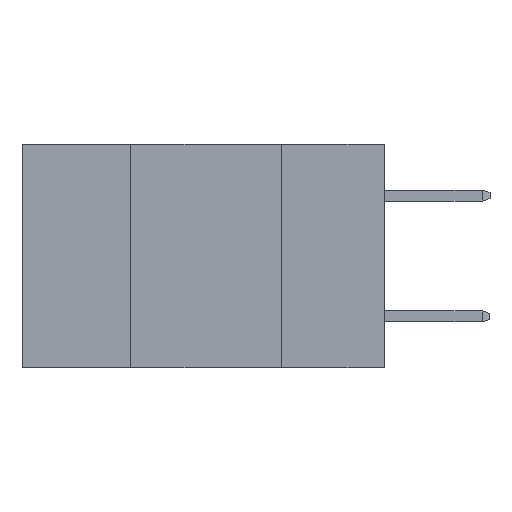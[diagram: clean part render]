
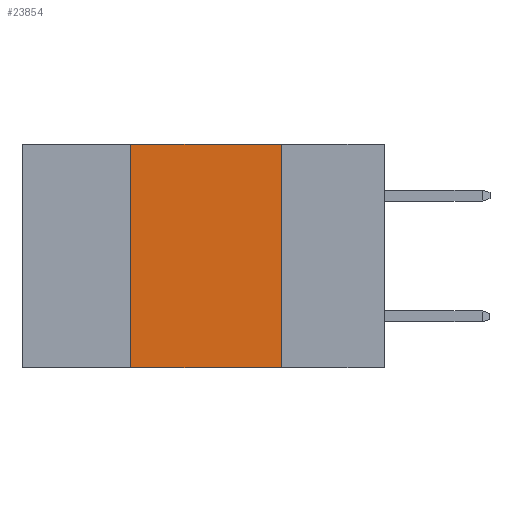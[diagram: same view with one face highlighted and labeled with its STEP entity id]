
A CAD part, left-side view. The second image highlights one B-rep face of the part: STEP entity #23854.
In plain terms, the highlighted planar face has unit normal (-1, 0, 0).
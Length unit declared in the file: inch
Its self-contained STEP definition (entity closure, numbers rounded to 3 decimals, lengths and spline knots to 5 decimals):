
#1426 = AXIS2_PLACEMENT_3D ( 'NONE', #3676, #22926, #11557 ) ;
#3478 = ORIENTED_EDGE ( 'NONE', *, *, #15090, .F. ) ;
#3676 = CARTESIAN_POINT ( 'NONE',  ( 0., 0.6, 0. ) ) ;
#3815 = DIRECTION ( 'NONE',  ( 0., 0., 1. ) ) ;
#3832 = LINE ( 'NONE', #7844, #13610 ) ;
#4682 = VERTEX_POINT ( 'NONE', #17868 ) ;
#4720 = VERTEX_POINT ( 'NONE', #16121 ) ;
#5701 = VERTEX_POINT ( 'NONE', #13211 ) ;
#6736 = VECTOR ( 'NONE', #3815, 39.37008 ) ;
#7844 = CARTESIAN_POINT ( 'NONE',  ( 0., 0.6, -0.37 ) ) ;
#8350 = CARTESIAN_POINT ( 'NONE',  ( 0., 0.17, 0. ) ) ;
#8696 = EDGE_LOOP ( 'NONE', ( #3478, #14446, #9935, #15042 ) ) ;
#8722 = CARTESIAN_POINT ( 'NONE',  ( 0., 0.6, 0. ) ) ;
#9371 = VECTOR ( 'NONE', #10516, 39.37008 ) ;
#9935 = ORIENTED_EDGE ( 'NONE', *, *, #16327, .F. ) ;
#10516 = DIRECTION ( 'NONE',  ( 0., -1., 0. ) ) ;
#11557 = DIRECTION ( 'NONE',  ( 0., 0., -1. ) ) ;
#12498 = LINE ( 'NONE', #22907, #6736 ) ;
#12610 = CARTESIAN_POINT ( 'NONE',  ( 0., 0.17, 0. ) ) ;
#13194 = EDGE_CURVE ( 'NONE', #4682, #13758, #19526, .T. ) ;
#13211 = CARTESIAN_POINT ( 'NONE',  ( 0., 0.42, -0.37 ) ) ;
#13610 = VECTOR ( 'NONE', #23116, 39.37008 ) ;
#13758 = VERTEX_POINT ( 'NONE', #8350 ) ;
#14446 = ORIENTED_EDGE ( 'NONE', *, *, #13194, .F. ) ;
#15042 = ORIENTED_EDGE ( 'NONE', *, *, #18908, .T. ) ;
#15090 = EDGE_CURVE ( 'NONE', #13758, #4720, #20318, .T. ) ;
#15277 = VECTOR ( 'NONE', #23948, 39.37008 ) ;
#16121 = CARTESIAN_POINT ( 'NONE',  ( 0., 0.17, -0.37 ) ) ;
#16327 = EDGE_CURVE ( 'NONE', #5701, #4682, #12498, .T. ) ;
#17868 = CARTESIAN_POINT ( 'NONE',  ( 0., 0.42, 0. ) ) ;
#18908 = EDGE_CURVE ( 'NONE', #5701, #4720, #3832, .T. ) ;
#19146 = PLANE ( 'NONE',  #1426 ) ;
#19526 = LINE ( 'NONE', #8722, #9371 ) ;
#20318 = LINE ( 'NONE', #12610, #15277 ) ;
#20876 = FACE_OUTER_BOUND ( 'NONE', #8696, .T. ) ;
#22907 = CARTESIAN_POINT ( 'NONE',  ( 0., 0.42, 0. ) ) ;
#22926 = DIRECTION ( 'NONE',  ( 1., 0., 0. ) ) ;
#23116 = DIRECTION ( 'NONE',  ( 0., -1., 0. ) ) ;
#23854 = ADVANCED_FACE ( 'NONE', ( #20876 ), #19146, .F. ) ;
#23948 = DIRECTION ( 'NONE',  ( 0., 0., -1. ) ) ;
